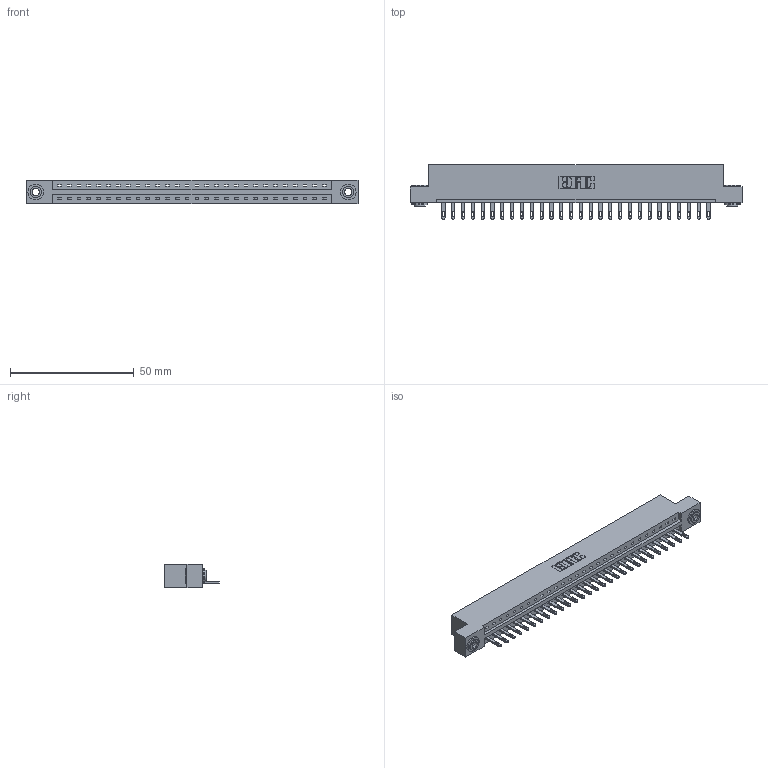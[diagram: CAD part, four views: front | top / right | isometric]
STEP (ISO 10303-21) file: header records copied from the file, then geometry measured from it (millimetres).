
FILE_DESCRIPTION (( 'STEP AP203' ), '1' );
FILE_NAME ('337-028-500-103.STEP', '2019-09-30T20:23:15', ( '' ), ( '' ), 'SwSTEP 2.0', 'SolidWorks 2016', '' );
FILE_SCHEMA (( 'CONFIG_CONTROL_DESIGN' ));
Length unit declared in the file: inch
Products named in the file (4): 345-292-001_345-293-100; 345-250-002_345-250-002-102; 337 Part_Flush Mounting Lugs - 0.156 Dia-TH; 337-028-500-103
Assembly tree (31 placements, depth 2):
  337-028-500-103
    337 Part_Flush Mounting Lugs - 0.156 Dia-TH
    345-292-001_345-293-100  x28
    345-250-002_345-250-002-102  x2
Bounding box: 133.96 x 21.85 x 9.4 mm (x, y, z)
Volume: 13784.4 mm3; surface area: 14464.5 mm2
Topology: 31 solids, 31 shells, 1776 faces, 5427 edges, 3614 vertices
Faces by surface type: plane 1200, cylinder 568, cone 8
Entity records: 23204 total; most frequent: CARTESIAN_POINT 4017, ORIENTED_EDGE 3974, DIRECTION 3445, EDGE_CURVE 1987, LINE 1831, VECTOR 1831, VERTEX_POINT 1322, AXIS2_PLACEMENT_3D 807
